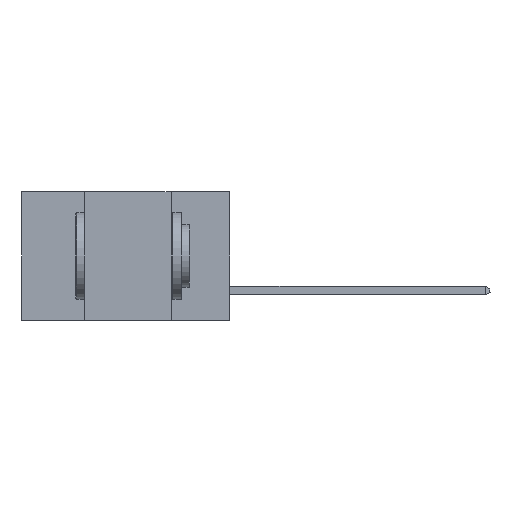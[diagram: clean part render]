
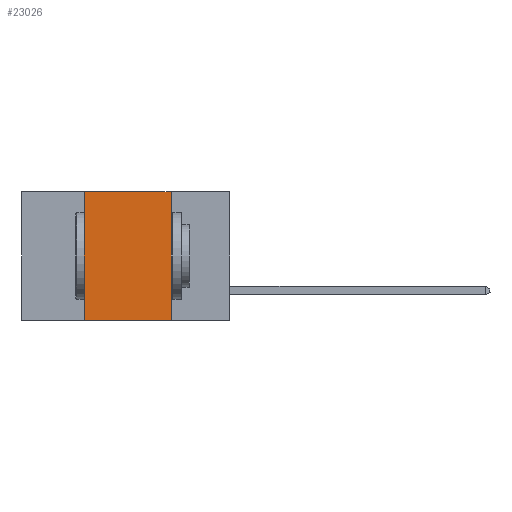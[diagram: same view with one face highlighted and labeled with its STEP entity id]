
A CAD part, left-side view. The second image highlights one B-rep face of the part: STEP entity #23026.
In plain terms, the highlighted planar face has unit normal (-1, 0, 0).
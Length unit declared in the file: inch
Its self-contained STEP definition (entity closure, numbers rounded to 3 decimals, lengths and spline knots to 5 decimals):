
#872 = ORIENTED_EDGE ( 'NONE', *, *, #3466, .F. ) ;
#914 = LINE ( 'NONE', #10193, #2534 ) ;
#1308 = DIRECTION ( 'NONE',  ( 0., 0., 1. ) ) ;
#2534 = VECTOR ( 'NONE', #26705, 39.37008 ) ;
#3122 = LINE ( 'NONE', #11794, #24555 ) ;
#3466 = EDGE_CURVE ( 'NONE', #6357, #9393, #3122, .T. ) ;
#4845 = LINE ( 'NONE', #11466, #10939 ) ;
#5023 = ORIENTED_EDGE ( 'NONE', *, *, #11440, .F. ) ;
#5545 = EDGE_CURVE ( 'NONE', #9393, #5784, #11861, .T. ) ;
#5687 = VECTOR ( 'NONE', #14713, 39.37008 ) ;
#5734 = CARTESIAN_POINT ( 'NONE',  ( 0., 0.6, 0. ) ) ;
#5784 = VERTEX_POINT ( 'NONE', #17536 ) ;
#6357 = VERTEX_POINT ( 'NONE', #15603 ) ;
#6382 = CARTESIAN_POINT ( 'NONE',  ( 0., 0.42, -0.37 ) ) ;
#7633 = DIRECTION ( 'NONE',  ( 0., -1., 0. ) ) ;
#7918 = PLANE ( 'NONE',  #11585 ) ;
#9023 = EDGE_LOOP ( 'NONE', ( #23354, #872, #5023, #25258 ) ) ;
#9393 = VERTEX_POINT ( 'NONE', #19605 ) ;
#9604 = EDGE_CURVE ( 'NONE', #19200, #5784, #914, .T. ) ;
#10193 = CARTESIAN_POINT ( 'NONE',  ( 0., 0.6, -0.37 ) ) ;
#10939 = VECTOR ( 'NONE', #1308, 39.37008 ) ;
#11440 = EDGE_CURVE ( 'NONE', #19200, #6357, #4845, .T. ) ;
#11466 = CARTESIAN_POINT ( 'NONE',  ( 0., 0.42, 0. ) ) ;
#11585 = AXIS2_PLACEMENT_3D ( 'NONE', #5734, #22370, #11908 ) ;
#11794 = CARTESIAN_POINT ( 'NONE',  ( 0., 0.6, 0. ) ) ;
#11861 = LINE ( 'NONE', #12541, #5687 ) ;
#11908 = DIRECTION ( 'NONE',  ( 0., 0., -1. ) ) ;
#12469 = FACE_OUTER_BOUND ( 'NONE', #9023, .T. ) ;
#12541 = CARTESIAN_POINT ( 'NONE',  ( 0., 0.17, 0. ) ) ;
#14713 = DIRECTION ( 'NONE',  ( 0., 0., -1. ) ) ;
#15603 = CARTESIAN_POINT ( 'NONE',  ( 0., 0.42, 0. ) ) ;
#17536 = CARTESIAN_POINT ( 'NONE',  ( 0., 0.17, -0.37 ) ) ;
#19200 = VERTEX_POINT ( 'NONE', #6382 ) ;
#19605 = CARTESIAN_POINT ( 'NONE',  ( 0., 0.17, 0. ) ) ;
#22370 = DIRECTION ( 'NONE',  ( 1., 0., 0. ) ) ;
#23026 = ADVANCED_FACE ( 'NONE', ( #12469 ), #7918, .F. ) ;
#23354 = ORIENTED_EDGE ( 'NONE', *, *, #5545, .F. ) ;
#24555 = VECTOR ( 'NONE', #7633, 39.37008 ) ;
#25258 = ORIENTED_EDGE ( 'NONE', *, *, #9604, .T. ) ;
#26705 = DIRECTION ( 'NONE',  ( 0., -1., 0. ) ) ;
